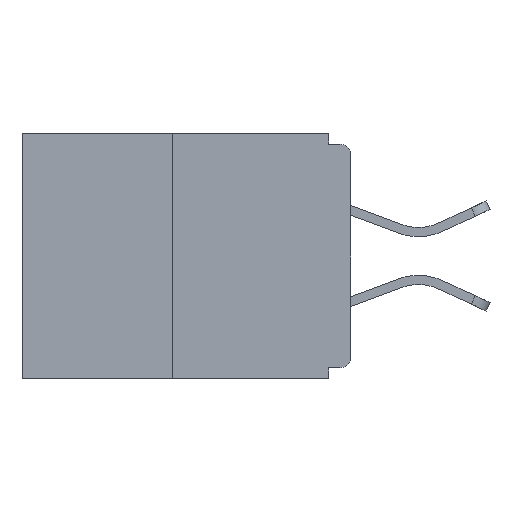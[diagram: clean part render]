
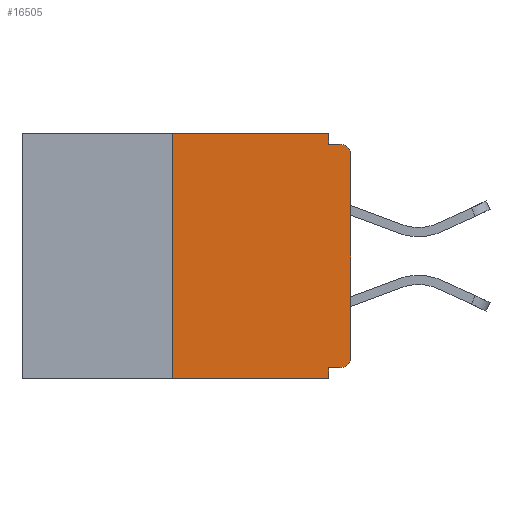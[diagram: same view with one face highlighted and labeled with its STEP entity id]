
A CAD part, left-side view. The second image highlights one B-rep face of the part: STEP entity #16505.
In plain terms, the highlighted planar face has unit normal (-1, 0, 0).
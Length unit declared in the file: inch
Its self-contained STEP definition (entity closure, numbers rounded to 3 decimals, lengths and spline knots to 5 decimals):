
#214 = EDGE_CURVE ( 'NONE', #17575, #17459, #10975, .T. ) ;
#385 = LINE ( 'NONE', #17188, #10408 ) ;
#443 = LINE ( 'NONE', #2596, #9046 ) ;
#571 = DIRECTION ( 'NONE',  ( 0., -1., 0. ) ) ;
#774 = EDGE_CURVE ( 'NONE', #12076, #2658, #2643, .T. ) ;
#1334 = FACE_OUTER_BOUND ( 'NONE', #10594, .T. ) ;
#1367 = ORIENTED_EDGE ( 'NONE', *, *, #774, .F. ) ;
#2177 = AXIS2_PLACEMENT_3D ( 'NONE', #19407, #8569, #23092 ) ;
#2596 = CARTESIAN_POINT ( 'NONE',  ( 0., 0., 0. ) ) ;
#2626 = DIRECTION ( 'NONE',  ( 0., 1., 0. ) ) ;
#2643 = LINE ( 'NONE', #5175, #13757 ) ;
#2658 = VERTEX_POINT ( 'NONE', #15330 ) ;
#2781 = CARTESIAN_POINT ( 'NONE',  ( 0., 0.031, 0. ) ) ;
#3131 = ORIENTED_EDGE ( 'NONE', *, *, #3582, .T. ) ;
#3159 = EDGE_CURVE ( 'NONE', #6826, #9152, #20148, .T. ) ;
#3190 = DIRECTION ( 'NONE',  ( 1., 0., 0. ) ) ;
#3209 = CARTESIAN_POINT ( 'NONE',  ( 0., 0., -0.313 ) ) ;
#3212 = ORIENTED_EDGE ( 'NONE', *, *, #214, .F. ) ;
#3582 = EDGE_CURVE ( 'NONE', #15166, #14530, #7368, .T. ) ;
#3868 = VECTOR ( 'NONE', #10471, 39.37008 ) ;
#4356 = ORIENTED_EDGE ( 'NONE', *, *, #7498, .F. ) ;
#4548 = DIRECTION ( 'NONE',  ( 0., 0., 1. ) ) ;
#4588 = DIRECTION ( 'NONE',  ( 0., 0., -1. ) ) ;
#4871 = ORIENTED_EDGE ( 'NONE', *, *, #7852, .T. ) ;
#5106 = DIRECTION ( 'NONE',  ( 0., 0., -1. ) ) ;
#5175 = CARTESIAN_POINT ( 'NONE',  ( 0., 0.46, 0. ) ) ;
#5482 = CARTESIAN_POINT ( 'NONE',  ( 0., 0.031, -0.015 ) ) ;
#5728 = ORIENTED_EDGE ( 'NONE', *, *, #18426, .T. ) ;
#5793 = LINE ( 'NONE', #11748, #21710 ) ;
#6162 = CARTESIAN_POINT ( 'NONE',  ( 0., 0., -0.015 ) ) ;
#6193 = CARTESIAN_POINT ( 'NONE',  ( 0., 0.031, -0.343 ) ) ;
#6330 = EDGE_CURVE ( 'NONE', #15166, #12076, #385, .T. ) ;
#6773 = VERTEX_POINT ( 'NONE', #20321 ) ;
#6826 = VERTEX_POINT ( 'NONE', #7804 ) ;
#7368 = LINE ( 'NONE', #19433, #17588 ) ;
#7379 = DIRECTION ( 'NONE',  ( -1., 0., 0. ) ) ;
#7498 = EDGE_CURVE ( 'NONE', #2658, #17575, #10759, .T. ) ;
#7551 = ORIENTED_EDGE ( 'NONE', *, *, #13049, .F. ) ;
#7804 = CARTESIAN_POINT ( 'NONE',  ( 0., 0.015, -0.328 ) ) ;
#7832 = VECTOR ( 'NONE', #571, 39.37008 ) ;
#7837 = CIRCLE ( 'NONE', #9363, 0.015 ) ;
#7852 = EDGE_CURVE ( 'NONE', #9152, #6773, #443, .T. ) ;
#8544 = DIRECTION ( 'NONE',  ( 0., -1., 0. ) ) ;
#8569 = DIRECTION ( 'NONE',  ( -1., 0., 0. ) ) ;
#8593 = DIRECTION ( 'NONE',  ( 0., -1., 0. ) ) ;
#9046 = VECTOR ( 'NONE', #11954, 39.37008 ) ;
#9152 = VERTEX_POINT ( 'NONE', #3209 ) ;
#9363 = AXIS2_PLACEMENT_3D ( 'NONE', #22056, #7379, #20066 ) ;
#10408 = VECTOR ( 'NONE', #4548, 39.37008 ) ;
#10471 = DIRECTION ( 'NONE',  ( 0., 0., -1. ) ) ;
#10472 = CARTESIAN_POINT ( 'NONE',  ( 0., 0.25, 0. ) ) ;
#10594 = EDGE_LOOP ( 'NONE', ( #1367, #21284, #3131, #11537, #7551, #22215, #4871, #5728, #3212, #4356 ) ) ;
#10759 = LINE ( 'NONE', #2781, #3868 ) ;
#10902 = LINE ( 'NONE', #6193, #17672 ) ;
#10975 = LINE ( 'NONE', #6162, #7832 ) ;
#11008 = EDGE_CURVE ( 'NONE', #21428, #14530, #10902, .T. ) ;
#11537 = ORIENTED_EDGE ( 'NONE', *, *, #11008, .F. ) ;
#11748 = CARTESIAN_POINT ( 'NONE',  ( 0., 0., -0.328 ) ) ;
#11954 = DIRECTION ( 'NONE',  ( 0., 0., 1. ) ) ;
#12076 = VERTEX_POINT ( 'NONE', #10472 ) ;
#13049 = EDGE_CURVE ( 'NONE', #6826, #21428, #5793, .T. ) ;
#13757 = VECTOR ( 'NONE', #8544, 39.37008 ) ;
#14179 = CARTESIAN_POINT ( 'NONE',  ( 0., 0.46, 0. ) ) ;
#14530 = VERTEX_POINT ( 'NONE', #23527 ) ;
#15166 = VERTEX_POINT ( 'NONE', #15430 ) ;
#15330 = CARTESIAN_POINT ( 'NONE',  ( 0., 0.031, 0. ) ) ;
#15430 = CARTESIAN_POINT ( 'NONE',  ( 0., 0.25, -0.343 ) ) ;
#16505 = ADVANCED_FACE ( 'NONE', ( #1334 ), #19397, .F. ) ;
#17188 = CARTESIAN_POINT ( 'NONE',  ( 0., 0.25, 0. ) ) ;
#17459 = VERTEX_POINT ( 'NONE', #17958 ) ;
#17575 = VERTEX_POINT ( 'NONE', #5482 ) ;
#17588 = VECTOR ( 'NONE', #8593, 39.37008 ) ;
#17672 = VECTOR ( 'NONE', #4588, 39.37008 ) ;
#17958 = CARTESIAN_POINT ( 'NONE',  ( 0., 0.015, -0.015 ) ) ;
#18426 = EDGE_CURVE ( 'NONE', #6773, #17459, #7837, .T. ) ;
#19397 = PLANE ( 'NONE',  #21007 ) ;
#19407 = CARTESIAN_POINT ( 'NONE',  ( 0., 0.015, -0.313 ) ) ;
#19433 = CARTESIAN_POINT ( 'NONE',  ( 0., 0.46, -0.343 ) ) ;
#20066 = DIRECTION ( 'NONE',  ( 0., 0., -1. ) ) ;
#20148 = CIRCLE ( 'NONE', #2177, 0.015 ) ;
#20310 = CARTESIAN_POINT ( 'NONE',  ( 0., 0.031, -0.328 ) ) ;
#20321 = CARTESIAN_POINT ( 'NONE',  ( 0., 0., -0.03 ) ) ;
#21007 = AXIS2_PLACEMENT_3D ( 'NONE', #14179, #3190, #5106 ) ;
#21284 = ORIENTED_EDGE ( 'NONE', *, *, #6330, .F. ) ;
#21428 = VERTEX_POINT ( 'NONE', #20310 ) ;
#21710 = VECTOR ( 'NONE', #2626, 39.37008 ) ;
#22056 = CARTESIAN_POINT ( 'NONE',  ( 0., 0.015, -0.03 ) ) ;
#22215 = ORIENTED_EDGE ( 'NONE', *, *, #3159, .T. ) ;
#23092 = DIRECTION ( 'NONE',  ( 0., 0., -1. ) ) ;
#23527 = CARTESIAN_POINT ( 'NONE',  ( 0., 0.031, -0.343 ) ) ;
